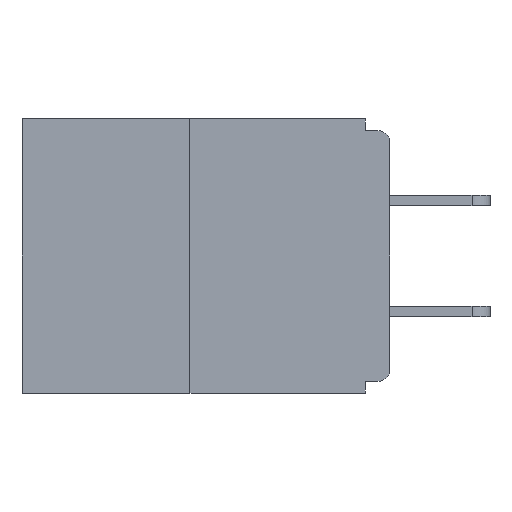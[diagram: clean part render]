
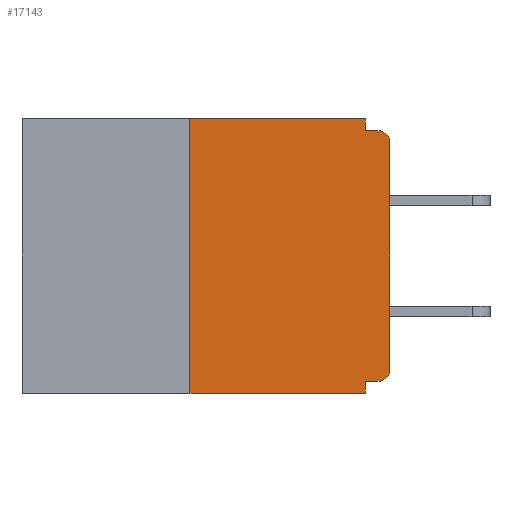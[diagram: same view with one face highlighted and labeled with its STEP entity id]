
A CAD part, left-side view. The second image highlights one B-rep face of the part: STEP entity #17143.
In plain terms, the highlighted planar face has unit normal (-1, 0, 0).
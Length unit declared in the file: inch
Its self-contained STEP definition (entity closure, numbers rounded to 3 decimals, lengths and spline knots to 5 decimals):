
#83 = AXIS2_PLACEMENT_3D ( 'NONE', #1265, #8193, #2726 ) ;
#534 = VERTEX_POINT ( 'NONE', #8796 ) ;
#593 = VERTEX_POINT ( 'NONE', #5454 ) ;
#771 = EDGE_LOOP ( 'NONE', ( #10465, #12490, #15881, #11981, #7565, #14447, #15615, #2207, #19247, #2968 ) ) ;
#1265 = CARTESIAN_POINT ( 'NONE',  ( 0., 0.015, -0.313 ) ) ;
#1594 = VECTOR ( 'NONE', #17335, 39.37008 ) ;
#1905 = CARTESIAN_POINT ( 'NONE',  ( 0., 0., -0.313 ) ) ;
#2207 = ORIENTED_EDGE ( 'NONE', *, *, #21515, .T. ) ;
#2644 = AXIS2_PLACEMENT_3D ( 'NONE', #10693, #8951, #10522 ) ;
#2726 = DIRECTION ( 'NONE',  ( 0., 0., -1. ) ) ;
#2962 = VERTEX_POINT ( 'NONE', #14872 ) ;
#2968 = ORIENTED_EDGE ( 'NONE', *, *, #21654, .F. ) ;
#3597 = CARTESIAN_POINT ( 'NONE',  ( 0., 0.031, -0.015 ) ) ;
#4557 = DIRECTION ( 'NONE',  ( 0., 0., 1. ) ) ;
#5454 = CARTESIAN_POINT ( 'NONE',  ( 0., 0.031, 0. ) ) ;
#5554 = VERTEX_POINT ( 'NONE', #12131 ) ;
#6063 = CARTESIAN_POINT ( 'NONE',  ( 0., 0.25, 0. ) ) ;
#6879 = PLANE ( 'NONE',  #2644 ) ;
#7175 = CARTESIAN_POINT ( 'NONE',  ( 0., 0., -0.015 ) ) ;
#7403 = LINE ( 'NONE', #14179, #18176 ) ;
#7565 = ORIENTED_EDGE ( 'NONE', *, *, #12255, .F. ) ;
#8193 = DIRECTION ( 'NONE',  ( -1., 0., 0. ) ) ;
#8198 = EDGE_CURVE ( 'NONE', #16991, #13663, #9376, .T. ) ;
#8304 = DIRECTION ( 'NONE',  ( -1., 0., 0. ) ) ;
#8372 = CARTESIAN_POINT ( 'NONE',  ( 0., 0.25, -0.343 ) ) ;
#8499 = EDGE_CURVE ( 'NONE', #21534, #18454, #20724, .T. ) ;
#8596 = FACE_OUTER_BOUND ( 'NONE', #771, .T. ) ;
#8720 = EDGE_CURVE ( 'NONE', #14971, #5554, #11076, .T. ) ;
#8796 = CARTESIAN_POINT ( 'NONE',  ( 0., 0., -0.03 ) ) ;
#8910 = CARTESIAN_POINT ( 'NONE',  ( 0., 0.031, 0. ) ) ;
#8951 = DIRECTION ( 'NONE',  ( 1., 0., 0. ) ) ;
#9156 = DIRECTION ( 'NONE',  ( 0., 0., -1. ) ) ;
#9376 = CIRCLE ( 'NONE', #83, 0.015 ) ;
#9829 = LINE ( 'NONE', #18855, #1594 ) ;
#10189 = VECTOR ( 'NONE', #10831, 39.37008 ) ;
#10465 = ORIENTED_EDGE ( 'NONE', *, *, #13652, .F. ) ;
#10522 = DIRECTION ( 'NONE',  ( 0., 0., -1. ) ) ;
#10693 = CARTESIAN_POINT ( 'NONE',  ( 0., 0.46, 0. ) ) ;
#10831 = DIRECTION ( 'NONE',  ( 0., -1., 0. ) ) ;
#11030 = CARTESIAN_POINT ( 'NONE',  ( 0., 0.031, -0.343 ) ) ;
#11076 = LINE ( 'NONE', #7175, #10189 ) ;
#11310 = DIRECTION ( 'NONE',  ( 0., 1., 0. ) ) ;
#11375 = EDGE_CURVE ( 'NONE', #21534, #13755, #19486, .T. ) ;
#11385 = EDGE_CURVE ( 'NONE', #2962, #13755, #9829, .T. ) ;
#11700 = VECTOR ( 'NONE', #11310, 39.37008 ) ;
#11961 = CARTESIAN_POINT ( 'NONE',  ( 0., 0.015, -0.328 ) ) ;
#11981 = ORIENTED_EDGE ( 'NONE', *, *, #11385, .F. ) ;
#12131 = CARTESIAN_POINT ( 'NONE',  ( 0., 0.015, -0.015 ) ) ;
#12255 = EDGE_CURVE ( 'NONE', #16991, #2962, #21662, .T. ) ;
#12490 = ORIENTED_EDGE ( 'NONE', *, *, #8499, .F. ) ;
#12507 = VECTOR ( 'NONE', #17907, 39.37008 ) ;
#13199 = EDGE_CURVE ( 'NONE', #13663, #534, #7403, .T. ) ;
#13652 = EDGE_CURVE ( 'NONE', #18454, #593, #19281, .T. ) ;
#13663 = VERTEX_POINT ( 'NONE', #1905 ) ;
#13703 = DIRECTION ( 'NONE',  ( 0., 0., -1. ) ) ;
#13755 = VERTEX_POINT ( 'NONE', #11030 ) ;
#13773 = CARTESIAN_POINT ( 'NONE',  ( 0., 0.015, -0.03 ) ) ;
#14179 = CARTESIAN_POINT ( 'NONE',  ( 0., 0., 0. ) ) ;
#14447 = ORIENTED_EDGE ( 'NONE', *, *, #8198, .T. ) ;
#14462 = VECTOR ( 'NONE', #9156, 39.37008 ) ;
#14872 = CARTESIAN_POINT ( 'NONE',  ( 0., 0.031, -0.328 ) ) ;
#14971 = VERTEX_POINT ( 'NONE', #3597 ) ;
#15533 = CARTESIAN_POINT ( 'NONE',  ( 0., 0.25, 0. ) ) ;
#15615 = ORIENTED_EDGE ( 'NONE', *, *, #13199, .T. ) ;
#15842 = CARTESIAN_POINT ( 'NONE',  ( 0., 0.46, -0.343 ) ) ;
#15881 = ORIENTED_EDGE ( 'NONE', *, *, #11375, .T. ) ;
#16180 = CARTESIAN_POINT ( 'NONE',  ( 0., 0.46, 0. ) ) ;
#16600 = AXIS2_PLACEMENT_3D ( 'NONE', #13773, #8304, #13703 ) ;
#16991 = VERTEX_POINT ( 'NONE', #11961 ) ;
#17143 = ADVANCED_FACE ( 'NONE', ( #8596 ), #6879, .F. ) ;
#17335 = DIRECTION ( 'NONE',  ( 0., 0., -1. ) ) ;
#17907 = DIRECTION ( 'NONE',  ( 0., -1., 0. ) ) ;
#18176 = VECTOR ( 'NONE', #23059, 39.37008 ) ;
#18428 = CIRCLE ( 'NONE', #16600, 0.015 ) ;
#18454 = VERTEX_POINT ( 'NONE', #15533 ) ;
#18855 = CARTESIAN_POINT ( 'NONE',  ( 0., 0.031, -0.343 ) ) ;
#18906 = VECTOR ( 'NONE', #19485, 39.37008 ) ;
#18989 = VECTOR ( 'NONE', #4557, 39.37008 ) ;
#19247 = ORIENTED_EDGE ( 'NONE', *, *, #8720, .F. ) ;
#19281 = LINE ( 'NONE', #16180, #12507 ) ;
#19485 = DIRECTION ( 'NONE',  ( 0., -1., 0. ) ) ;
#19486 = LINE ( 'NONE', #15842, #18906 ) ;
#19563 = LINE ( 'NONE', #8910, #14462 ) ;
#20724 = LINE ( 'NONE', #6063, #18989 ) ;
#21515 = EDGE_CURVE ( 'NONE', #534, #5554, #18428, .T. ) ;
#21534 = VERTEX_POINT ( 'NONE', #8372 ) ;
#21654 = EDGE_CURVE ( 'NONE', #593, #14971, #19563, .T. ) ;
#21662 = LINE ( 'NONE', #22017, #11700 ) ;
#22017 = CARTESIAN_POINT ( 'NONE',  ( 0., 0., -0.328 ) ) ;
#23059 = DIRECTION ( 'NONE',  ( 0., 0., 1. ) ) ;
